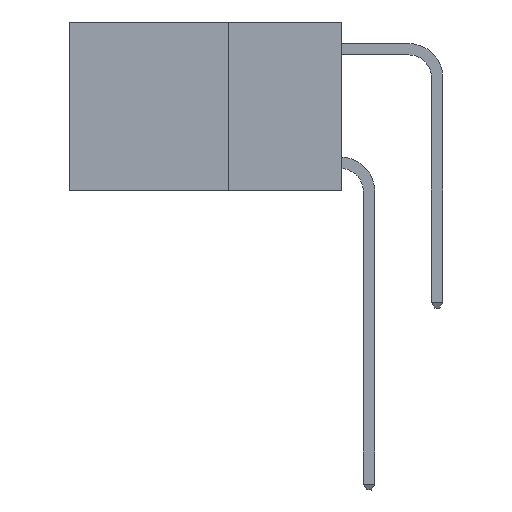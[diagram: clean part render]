
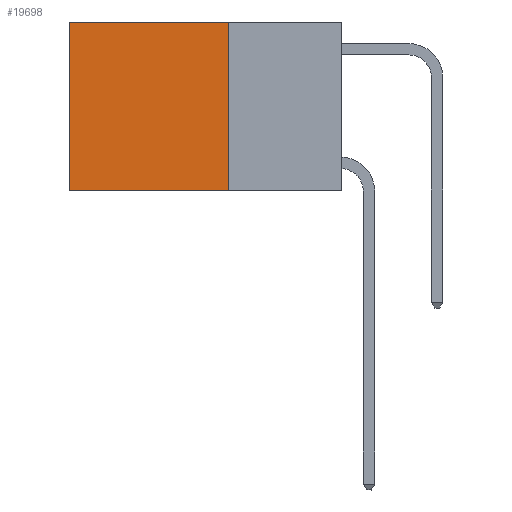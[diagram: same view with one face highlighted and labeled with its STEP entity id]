
A CAD part, left-side view. The second image highlights one B-rep face of the part: STEP entity #19698.
In plain terms, the highlighted planar face has unit normal (-1, 0, 0).
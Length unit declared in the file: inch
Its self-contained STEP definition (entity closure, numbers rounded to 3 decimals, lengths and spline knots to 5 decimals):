
#287 = VECTOR ( 'NONE', #14156, 39.37008 ) ;
#923 = CARTESIAN_POINT ( 'NONE',  ( 0.2625, 0.25, -0.37 ) ) ;
#1218 = PLANE ( 'NONE',  #23531 ) ;
#1782 = CARTESIAN_POINT ( 'NONE',  ( 0.2625, 0.6, -0.37 ) ) ;
#1914 = EDGE_LOOP ( 'NONE', ( #9740, #25957, #19734, #26380 ) ) ;
#3354 = CARTESIAN_POINT ( 'NONE',  ( 0.2625, 0.6, 0. ) ) ;
#4574 = CARTESIAN_POINT ( 'NONE',  ( 0.2625, 0.25, 0. ) ) ;
#5340 = FACE_OUTER_BOUND ( 'NONE', #1914, .T. ) ;
#7267 = DIRECTION ( 'NONE',  ( 0., 1., 0. ) ) ;
#8288 = EDGE_CURVE ( 'NONE', #17846, #20914, #9464, .T. ) ;
#9316 = DIRECTION ( 'NONE',  ( 0., 0., -1. ) ) ;
#9464 = LINE ( 'NONE', #4574, #10537 ) ;
#9740 = ORIENTED_EDGE ( 'NONE', *, *, #12881, .T. ) ;
#9770 = CARTESIAN_POINT ( 'NONE',  ( 0.2625, 0.25, -0.37 ) ) ;
#10537 = VECTOR ( 'NONE', #7267, 39.37008 ) ;
#11453 = EDGE_CURVE ( 'NONE', #13610, #17567, #16102, .T. ) ;
#12881 = EDGE_CURVE ( 'NONE', #20914, #17567, #19976, .T. ) ;
#13572 = DIRECTION ( 'NONE',  ( 0., 0., -1. ) ) ;
#13610 = VERTEX_POINT ( 'NONE', #923 ) ;
#13836 = CARTESIAN_POINT ( 'NONE',  ( 0.2625, 0.25, 0. ) ) ;
#14156 = DIRECTION ( 'NONE',  ( 0., 1., 0. ) ) ;
#15516 = LINE ( 'NONE', #24140, #25734 ) ;
#16102 = LINE ( 'NONE', #9770, #287 ) ;
#16464 = EDGE_CURVE ( 'NONE', #17846, #13610, #15516, .T. ) ;
#17567 = VERTEX_POINT ( 'NONE', #1782 ) ;
#17846 = VERTEX_POINT ( 'NONE', #23066 ) ;
#18727 = CARTESIAN_POINT ( 'NONE',  ( 0.2625, 0.6, 0. ) ) ;
#19698 = ADVANCED_FACE ( 'NONE', ( #5340 ), #1218, .F. ) ;
#19734 = ORIENTED_EDGE ( 'NONE', *, *, #16464, .F. ) ;
#19841 = DIRECTION ( 'NONE',  ( 0., 0., -1. ) ) ;
#19976 = LINE ( 'NONE', #3354, #21755 ) ;
#20914 = VERTEX_POINT ( 'NONE', #18727 ) ;
#21755 = VECTOR ( 'NONE', #19841, 39.37008 ) ;
#23066 = CARTESIAN_POINT ( 'NONE',  ( 0.2625, 0.25, 0. ) ) ;
#23531 = AXIS2_PLACEMENT_3D ( 'NONE', #13836, #23880, #13572 ) ;
#23880 = DIRECTION ( 'NONE',  ( 1., 0., 0. ) ) ;
#24140 = CARTESIAN_POINT ( 'NONE',  ( 0.2625, 0.25, 0. ) ) ;
#25734 = VECTOR ( 'NONE', #9316, 39.37008 ) ;
#25957 = ORIENTED_EDGE ( 'NONE', *, *, #11453, .F. ) ;
#26380 = ORIENTED_EDGE ( 'NONE', *, *, #8288, .T. ) ;
